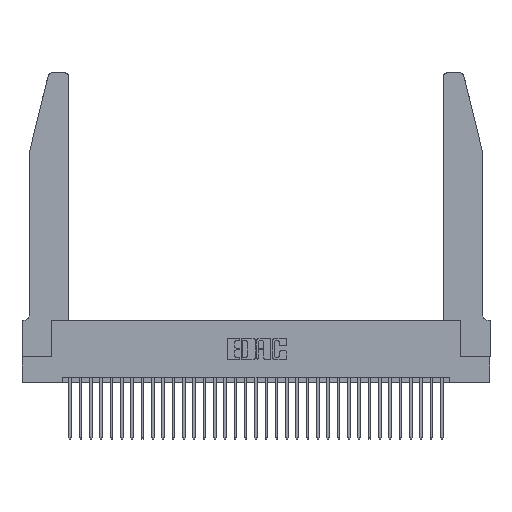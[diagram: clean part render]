
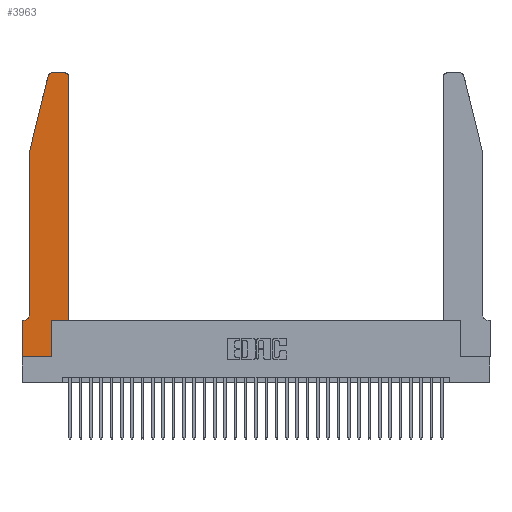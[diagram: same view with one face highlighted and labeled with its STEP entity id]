
A CAD part, top view. The second image highlights one B-rep face of the part: STEP entity #3963.
In plain terms, the highlighted planar face has unit normal (0, 0, 1).
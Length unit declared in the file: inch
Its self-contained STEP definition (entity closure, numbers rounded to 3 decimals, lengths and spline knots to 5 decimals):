
#558 = EDGE_CURVE ( 'NONE', #13626, #29490, #24957, .T. ) ;
#1018 = VERTEX_POINT ( 'NONE', #24183 ) ;
#1474 = EDGE_CURVE ( 'NONE', #34448, #24406, #21661, .T. ) ;
#1878 = LINE ( 'NONE', #11059, #22465 ) ;
#2171 = ORIENTED_EDGE ( 'NONE', *, *, #558, .T. ) ;
#2194 = DIRECTION ( 'NONE',  ( 1., 0., 0. ) ) ;
#2252 = DIRECTION ( 'NONE',  ( 0., 0., -1. ) ) ;
#2272 = ORIENTED_EDGE ( 'NONE', *, *, #5189, .T. ) ;
#2363 = ORIENTED_EDGE ( 'NONE', *, *, #22916, .T. ) ;
#2815 = ORIENTED_EDGE ( 'NONE', *, *, #24263, .T. ) ;
#2883 = DIRECTION ( 'NONE',  ( -1., 0., 0. ) ) ;
#3195 = ORIENTED_EDGE ( 'NONE', *, *, #1474, .T. ) ;
#3513 = PLANE ( 'NONE',  #16120 ) ;
#3618 = VECTOR ( 'NONE', #8823, 39.37008 ) ;
#3856 = EDGE_LOOP ( 'NONE', ( #2171, #2272, #2815, #2363, #5773, #7990, #3195, #5272, #14308, #14616, #22684, #17159 ) ) ;
#3929 = DIRECTION ( 'NONE',  ( 0., 1., 0. ) ) ;
#3963 = ADVANCED_FACE ( 'NONE', ( #18169 ), #3513, .T. ) ;
#4134 = CARTESIAN_POINT ( 'NONE',  ( 0.0055, 0.35, 0.37 ) ) ;
#4818 = AXIS2_PLACEMENT_3D ( 'NONE', #12028, #30464, #14711 ) ;
#4959 = VERTEX_POINT ( 'NONE', #6890 ) ;
#5189 = EDGE_CURVE ( 'NONE', #29490, #4959, #16852, .T. ) ;
#5272 = ORIENTED_EDGE ( 'NONE', *, *, #7274, .T. ) ;
#5773 = ORIENTED_EDGE ( 'NONE', *, *, #28763, .T. ) ;
#6087 = VERTEX_POINT ( 'NONE', #14019 ) ;
#6275 = EDGE_CURVE ( 'NONE', #29149, #29067, #31995, .T. ) ;
#6890 = CARTESIAN_POINT ( 'NONE',  ( 0.25487, 2.72718, 0.37 ) ) ;
#7274 = EDGE_CURVE ( 'NONE', #24406, #31866, #23819, .T. ) ;
#7696 = CARTESIAN_POINT ( 'NONE',  ( 0., 0., 0.37 ) ) ;
#7990 = ORIENTED_EDGE ( 'NONE', *, *, #24156, .T. ) ;
#8247 = VECTOR ( 'NONE', #13640, 39.37008 ) ;
#8823 = DIRECTION ( 'NONE',  ( -1., 0., 0. ) ) ;
#9008 = VECTOR ( 'NONE', #32924, 39.37008 ) ;
#9212 = AXIS2_PLACEMENT_3D ( 'NONE', #18351, #2252, #21023 ) ;
#9288 = CARTESIAN_POINT ( 'NONE',  ( 0.4505, 0.35, 0.37 ) ) ;
#11059 = CARTESIAN_POINT ( 'NONE',  ( 0.2865, 0.35, 0.37 ) ) ;
#12013 = CARTESIAN_POINT ( 'NONE',  ( 0.4505, 0.35, 0.37 ) ) ;
#12028 = CARTESIAN_POINT ( 'NONE',  ( 0.4205, 2.72, 0.37 ) ) ;
#12361 = VECTOR ( 'NONE', #2883, 39.37008 ) ;
#13271 = EDGE_CURVE ( 'NONE', #31866, #6087, #1878, .T. ) ;
#13626 = VERTEX_POINT ( 'NONE', #23248 ) ;
#13640 = DIRECTION ( 'NONE',  ( 0., -1., 0. ) ) ;
#14019 = CARTESIAN_POINT ( 'NONE',  ( 0.2865, 0.35, 0.37 ) ) ;
#14308 = ORIENTED_EDGE ( 'NONE', *, *, #13271, .T. ) ;
#14409 = CARTESIAN_POINT ( 'NONE',  ( 0., 0.35, 0.37 ) ) ;
#14560 = CARTESIAN_POINT ( 'NONE',  ( 0.4505, 0.35, 0.37 ) ) ;
#14616 = ORIENTED_EDGE ( 'NONE', *, *, #24953, .T. ) ;
#14711 = DIRECTION ( 'NONE',  ( 1., 0., 0. ) ) ;
#15502 = VECTOR ( 'NONE', #26133, 39.37008 ) ;
#15819 = CARTESIAN_POINT ( 'NONE',  ( 0.284, 2.72, 0.37 ) ) ;
#16082 = VERTEX_POINT ( 'NONE', #4134 ) ;
#16120 = AXIS2_PLACEMENT_3D ( 'NONE', #14409, #32783, #17034 ) ;
#16298 = CARTESIAN_POINT ( 'NONE',  ( 0.0755, 2., 0.37 ) ) ;
#16346 = CARTESIAN_POINT ( 'NONE',  ( 0.0755, 0.35, 0.37 ) ) ;
#16852 = CIRCLE ( 'NONE', #28239, 0.03 ) ;
#16909 = LINE ( 'NONE', #30004, #29287 ) ;
#17034 = DIRECTION ( 'NONE',  ( 1., 0., 0. ) ) ;
#17159 = ORIENTED_EDGE ( 'NONE', *, *, #26363, .T. ) ;
#18169 = FACE_OUTER_BOUND ( 'NONE', #3856, .T. ) ;
#18351 = CARTESIAN_POINT ( 'NONE',  ( 0.0055, 0.42, 0.37 ) ) ;
#18419 = DIRECTION ( 'NONE',  ( 1., 0., 0. ) ) ;
#18478 = CARTESIAN_POINT ( 'NONE',  ( 0.2605, 2.75, 0.37 ) ) ;
#19138 = CARTESIAN_POINT ( 'NONE',  ( 0.284, 2.75, 0.37 ) ) ;
#19395 = LINE ( 'NONE', #16346, #12361 ) ;
#20460 = CIRCLE ( 'NONE', #9212, 0.07 ) ;
#21023 = DIRECTION ( 'NONE',  ( -1., 0., 0. ) ) ;
#21661 = LINE ( 'NONE', #25686, #15502 ) ;
#22205 = CIRCLE ( 'NONE', #4818, 0.03 ) ;
#22214 = DIRECTION ( 'NONE',  ( -0.239, -0.971, 0. ) ) ;
#22465 = VECTOR ( 'NONE', #32138, 39.37008 ) ;
#22684 = ORIENTED_EDGE ( 'NONE', *, *, #6275, .T. ) ;
#22916 = EDGE_CURVE ( 'NONE', #1018, #31309, #29383, .T. ) ;
#23248 = CARTESIAN_POINT ( 'NONE',  ( 0.4205, 2.75, 0.37 ) ) ;
#23819 = LINE ( 'NONE', #7696, #29938 ) ;
#23959 = CARTESIAN_POINT ( 'NONE',  ( 0.2865, 0., 0.37 ) ) ;
#23982 = LINE ( 'NONE', #14560, #9008 ) ;
#24156 = EDGE_CURVE ( 'NONE', #16082, #34448, #19395, .T. ) ;
#24183 = CARTESIAN_POINT ( 'NONE',  ( 0.0755, 2., 0.37 ) ) ;
#24263 = EDGE_CURVE ( 'NONE', #4959, #1018, #16909, .T. ) ;
#24406 = VERTEX_POINT ( 'NONE', #25660 ) ;
#24844 = CARTESIAN_POINT ( 'NONE',  ( 0.4505, 2.72, 0.37 ) ) ;
#24953 = EDGE_CURVE ( 'NONE', #6087, #29149, #23982, .T. ) ;
#24957 = LINE ( 'NONE', #18478, #3618 ) ;
#25049 = VECTOR ( 'NONE', #3929, 39.37008 ) ;
#25660 = CARTESIAN_POINT ( 'NONE',  ( 0., 0., 0.37 ) ) ;
#25686 = CARTESIAN_POINT ( 'NONE',  ( 0., 0., 0.37 ) ) ;
#26133 = DIRECTION ( 'NONE',  ( 0., -1., 0. ) ) ;
#26363 = EDGE_CURVE ( 'NONE', #29067, #13626, #22205, .T. ) ;
#26715 = CARTESIAN_POINT ( 'NONE',  ( 0.0755, 0.42, 0.37 ) ) ;
#28239 = AXIS2_PLACEMENT_3D ( 'NONE', #15819, #34140, #18419 ) ;
#28763 = EDGE_CURVE ( 'NONE', #31309, #16082, #20460, .T. ) ;
#29067 = VERTEX_POINT ( 'NONE', #24844 ) ;
#29149 = VERTEX_POINT ( 'NONE', #9288 ) ;
#29287 = VECTOR ( 'NONE', #22214, 39.37008 ) ;
#29383 = LINE ( 'NONE', #16298, #8247 ) ;
#29490 = VERTEX_POINT ( 'NONE', #19138 ) ;
#29938 = VECTOR ( 'NONE', #2194, 39.37008 ) ;
#30004 = CARTESIAN_POINT ( 'NONE',  ( 0.0755, 2., 0.37 ) ) ;
#30464 = DIRECTION ( 'NONE',  ( 0., 0., 1. ) ) ;
#30465 = CARTESIAN_POINT ( 'NONE',  ( 0., 0.35, 0.37 ) ) ;
#31309 = VERTEX_POINT ( 'NONE', #26715 ) ;
#31866 = VERTEX_POINT ( 'NONE', #23959 ) ;
#31995 = LINE ( 'NONE', #12013, #25049 ) ;
#32138 = DIRECTION ( 'NONE',  ( 0., 1., 0. ) ) ;
#32783 = DIRECTION ( 'NONE',  ( 0., 0., 1. ) ) ;
#32924 = DIRECTION ( 'NONE',  ( 1., 0., 0. ) ) ;
#34140 = DIRECTION ( 'NONE',  ( 0., 0., 1. ) ) ;
#34448 = VERTEX_POINT ( 'NONE', #30465 ) ;
